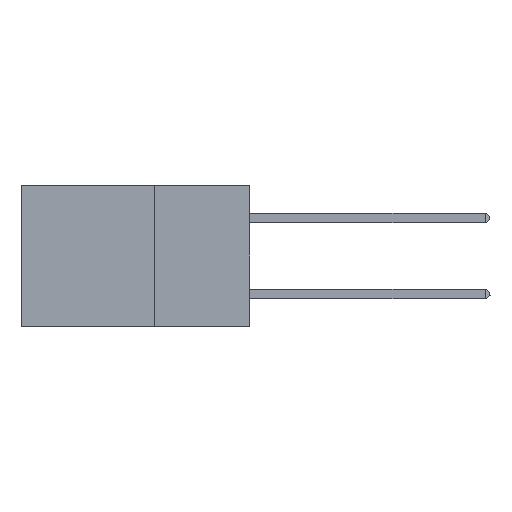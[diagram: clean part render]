
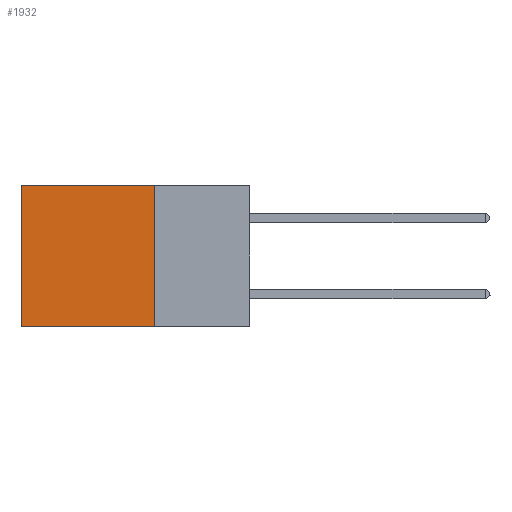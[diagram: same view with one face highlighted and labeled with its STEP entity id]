
A CAD part, left-side view. The second image highlights one B-rep face of the part: STEP entity #1932.
In plain terms, the highlighted planar face has unit normal (-1, 0, 0).
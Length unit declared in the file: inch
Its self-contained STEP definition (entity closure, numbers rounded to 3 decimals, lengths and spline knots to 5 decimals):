
#32 = CARTESIAN_POINT ( 'NONE',  ( 0.2875, 0.25, 0. ) ) ;
#1932 = ADVANCED_FACE ( 'NONE', ( #26988 ), #43676, .F. ) ;
#2308 = LINE ( 'NONE', #4998, #34578 ) ;
#4349 = ORIENTED_EDGE ( 'NONE', *, *, #12320, .T. ) ;
#4936 = CARTESIAN_POINT ( 'NONE',  ( 0.2875, 0.6, 0. ) ) ;
#4998 = CARTESIAN_POINT ( 'NONE',  ( 0.2875, 0.25, -0.37 ) ) ;
#5924 = CARTESIAN_POINT ( 'NONE',  ( 0.2875, 0.6, 0. ) ) ;
#6525 = DIRECTION ( 'NONE',  ( 0., 0., -1. ) ) ;
#8891 = VECTOR ( 'NONE', #12887, 39.37008 ) ;
#9908 = EDGE_CURVE ( 'NONE', #11162, #11998, #13092, .T. ) ;
#10385 = DIRECTION ( 'NONE',  ( 0., 0., -1. ) ) ;
#11162 = VERTEX_POINT ( 'NONE', #27818 ) ;
#11998 = VERTEX_POINT ( 'NONE', #13063 ) ;
#12320 = EDGE_CURVE ( 'NONE', #11162, #22651, #39591, .T. ) ;
#12887 = DIRECTION ( 'NONE',  ( 0., 0., -1. ) ) ;
#13063 = CARTESIAN_POINT ( 'NONE',  ( 0.2875, 0.25, -0.37 ) ) ;
#13085 = CARTESIAN_POINT ( 'NONE',  ( 0.2875, 0.6, -0.37 ) ) ;
#13092 = LINE ( 'NONE', #32, #19417 ) ;
#13486 = DIRECTION ( 'NONE',  ( 1., 0., 0. ) ) ;
#16030 = DIRECTION ( 'NONE',  ( 0., 1., 0. ) ) ;
#16440 = EDGE_CURVE ( 'NONE', #11998, #28967, #2308, .T. ) ;
#16613 = DIRECTION ( 'NONE',  ( 0., 1., 0. ) ) ;
#17115 = AXIS2_PLACEMENT_3D ( 'NONE', #40297, #13486, #6525 ) ;
#19417 = VECTOR ( 'NONE', #10385, 39.37008 ) ;
#22474 = CARTESIAN_POINT ( 'NONE',  ( 0.2875, 0.25, 0. ) ) ;
#22575 = EDGE_CURVE ( 'NONE', #22651, #28967, #33389, .T. ) ;
#22651 = VERTEX_POINT ( 'NONE', #4936 ) ;
#24403 = EDGE_LOOP ( 'NONE', ( #33235, #39350, #40852, #4349 ) ) ;
#26988 = FACE_OUTER_BOUND ( 'NONE', #24403, .T. ) ;
#27818 = CARTESIAN_POINT ( 'NONE',  ( 0.2875, 0.25, 0. ) ) ;
#28967 = VERTEX_POINT ( 'NONE', #13085 ) ;
#33235 = ORIENTED_EDGE ( 'NONE', *, *, #22575, .T. ) ;
#33389 = LINE ( 'NONE', #5924, #8891 ) ;
#34578 = VECTOR ( 'NONE', #16030, 39.37008 ) ;
#39350 = ORIENTED_EDGE ( 'NONE', *, *, #16440, .F. ) ;
#39591 = LINE ( 'NONE', #22474, #40127 ) ;
#40127 = VECTOR ( 'NONE', #16613, 39.37008 ) ;
#40297 = CARTESIAN_POINT ( 'NONE',  ( 0.2875, 0.25, 0. ) ) ;
#40852 = ORIENTED_EDGE ( 'NONE', *, *, #9908, .F. ) ;
#43676 = PLANE ( 'NONE',  #17115 ) ;
